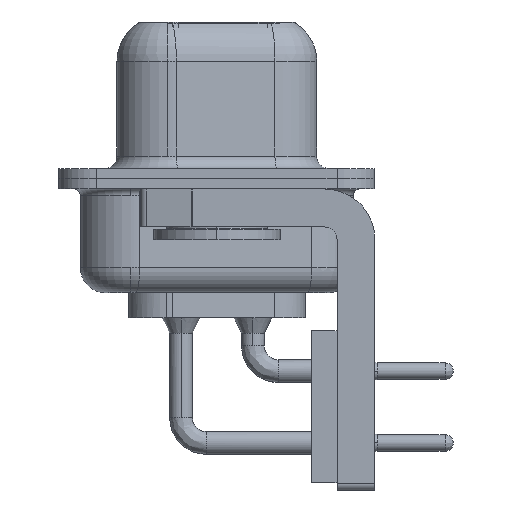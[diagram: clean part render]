
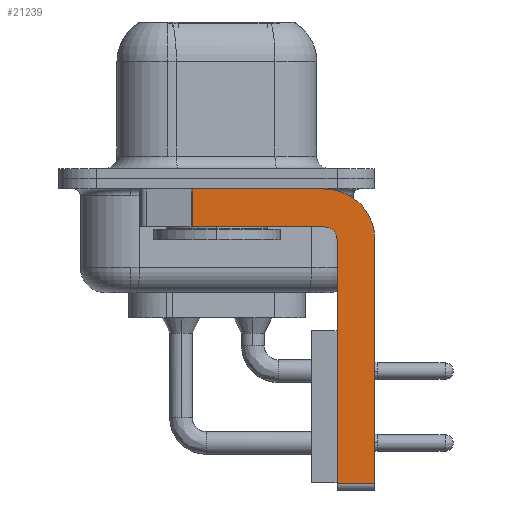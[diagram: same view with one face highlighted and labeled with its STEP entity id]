
A CAD part, left-side view. The second image highlights one B-rep face of the part: STEP entity #21239.
In plain terms, the highlighted planar face has unit normal (-1, 0, 0).
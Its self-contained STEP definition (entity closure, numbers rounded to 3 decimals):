
#61 = EDGE_CURVE ( 'NONE', #13793, #3360, #4816, .T. ) ;
#393 = ORIENTED_EDGE ( 'NONE', *, *, #61, .T. ) ;
#423 = DIRECTION ( 'NONE',  ( 1., 0., 0. ) ) ;
#534 = DIRECTION ( 'NONE',  ( 0., 0., -1. ) ) ;
#1154 = CARTESIAN_POINT ( 'NONE',  ( -2.9, 0.978, -1.9 ) ) ;
#1234 = ORIENTED_EDGE ( 'NONE', *, *, #21657, .F. ) ;
#1652 = CARTESIAN_POINT ( 'NONE',  ( -2.9, -6.25, -12.05 ) ) ;
#1697 = AXIS2_PLACEMENT_3D ( 'NONE', #14634, #2950, #16490 ) ;
#2386 = VECTOR ( 'NONE', #2713, 1000. ) ;
#2548 = VERTEX_POINT ( 'NONE', #20793 ) ;
#2713 = DIRECTION ( 'NONE',  ( 0., 0., 1. ) ) ;
#2915 = CARTESIAN_POINT ( 'NONE',  ( -2.9, -4.25, -1.9 ) ) ;
#2950 = DIRECTION ( 'NONE',  ( -1., 0., 0. ) ) ;
#3360 = VERTEX_POINT ( 'NONE', #1154 ) ;
#3460 = ORIENTED_EDGE ( 'NONE', *, *, #10310, .F. ) ;
#3591 = LINE ( 'NONE', #23923, #2386 ) ;
#4126 = VERTEX_POINT ( 'NONE', #22561 ) ;
#4303 = CARTESIAN_POINT ( 'NONE',  ( -2.9, 0.978, -0.4 ) ) ;
#4647 = VECTOR ( 'NONE', #534, 1000. ) ;
#4730 = EDGE_CURVE ( 'NONE', #20064, #3360, #20481, .T. ) ;
#4816 = LINE ( 'NONE', #22345, #24685 ) ;
#4904 = CARTESIAN_POINT ( 'NONE',  ( -2.9, -4.25, -2.4 ) ) ;
#5040 = VERTEX_POINT ( 'NONE', #22922 ) ;
#5066 = CIRCLE ( 'NONE', #5311, 2. ) ;
#5311 = AXIS2_PLACEMENT_3D ( 'NONE', #12179, #423, #14087 ) ;
#6488 = CARTESIAN_POINT ( 'NONE',  ( -2.9, -4.25, -12.05 ) ) ;
#6624 = VERTEX_POINT ( 'NONE', #19911 ) ;
#6702 = DIRECTION ( 'NONE',  ( 0., 1., 0. ) ) ;
#7469 = CIRCLE ( 'NONE', #1697, 0.5 ) ;
#7531 = ORIENTED_EDGE ( 'NONE', *, *, #8947, .F. ) ;
#8159 = CARTESIAN_POINT ( 'NONE',  ( -2.9, 3., -0.4 ) ) ;
#8947 = EDGE_CURVE ( 'NONE', #4126, #6624, #3591, .T. ) ;
#8955 = DIRECTION ( 'NONE',  ( 0., 0., -1. ) ) ;
#9201 = LINE ( 'NONE', #6488, #18729 ) ;
#9281 = LINE ( 'NONE', #23614, #4647 ) ;
#9599 = AXIS2_PLACEMENT_3D ( 'NONE', #4904, #20341, #8955 ) ;
#10053 = DIRECTION ( 'NONE',  ( 0., 0., -1. ) ) ;
#10310 = EDGE_CURVE ( 'NONE', #5040, #2548, #5066, .T. ) ;
#12132 = FACE_OUTER_BOUND ( 'NONE', #15062, .T. ) ;
#12179 = CARTESIAN_POINT ( 'NONE',  ( -2.9, -4.25, -2.4 ) ) ;
#12372 = DIRECTION ( 'NONE',  ( 0., -1., 0. ) ) ;
#13793 = VERTEX_POINT ( 'NONE', #4303 ) ;
#13887 = LINE ( 'NONE', #8159, #18274 ) ;
#14087 = DIRECTION ( 'NONE',  ( 0., 0., -1. ) ) ;
#14634 = CARTESIAN_POINT ( 'NONE',  ( -2.9, -4.25, -2.4 ) ) ;
#14771 = ORIENTED_EDGE ( 'NONE', *, *, #21184, .F. ) ;
#15062 = EDGE_LOOP ( 'NONE', ( #1234, #393, #21614, #14771, #7531, #24143, #15720, #3460 ) ) ;
#15720 = ORIENTED_EDGE ( 'NONE', *, *, #15893, .F. ) ;
#15893 = EDGE_CURVE ( 'NONE', #2548, #19602, #9281, .T. ) ;
#15897 = DIRECTION ( 'NONE',  ( 0., -1., 0. ) ) ;
#16490 = DIRECTION ( 'NONE',  ( 0., 0., 1. ) ) ;
#17579 = EDGE_CURVE ( 'NONE', #4126, #19602, #9201, .T. ) ;
#18274 = VECTOR ( 'NONE', #15897, 1000. ) ;
#18464 = PLANE ( 'NONE',  #9599 ) ;
#18729 = VECTOR ( 'NONE', #12372, 1000. ) ;
#19602 = VERTEX_POINT ( 'NONE', #1652 ) ;
#19911 = CARTESIAN_POINT ( 'NONE',  ( -2.9, -4.75, -2.4 ) ) ;
#20064 = VERTEX_POINT ( 'NONE', #20222 ) ;
#20222 = CARTESIAN_POINT ( 'NONE',  ( -2.9, -4.25, -1.9 ) ) ;
#20341 = DIRECTION ( 'NONE',  ( 1., 0., 0. ) ) ;
#20481 = LINE ( 'NONE', #2915, #21669 ) ;
#20793 = CARTESIAN_POINT ( 'NONE',  ( -2.9, -6.25, -2.4 ) ) ;
#21184 = EDGE_CURVE ( 'NONE', #6624, #20064, #7469, .T. ) ;
#21239 = ADVANCED_FACE ( 'NONE', ( #12132 ), #18464, .F. ) ;
#21614 = ORIENTED_EDGE ( 'NONE', *, *, #4730, .F. ) ;
#21657 = EDGE_CURVE ( 'NONE', #13793, #5040, #13887, .T. ) ;
#21669 = VECTOR ( 'NONE', #6702, 1000. ) ;
#22345 = CARTESIAN_POINT ( 'NONE',  ( -2.9, 0.978, -1.9 ) ) ;
#22561 = CARTESIAN_POINT ( 'NONE',  ( -2.9, -4.75, -12.05 ) ) ;
#22922 = CARTESIAN_POINT ( 'NONE',  ( -2.9, -4.25, -0.4 ) ) ;
#23614 = CARTESIAN_POINT ( 'NONE',  ( -2.9, -6.25, -2.4 ) ) ;
#23923 = CARTESIAN_POINT ( 'NONE',  ( -2.9, -4.75, -12.3 ) ) ;
#24143 = ORIENTED_EDGE ( 'NONE', *, *, #17579, .T. ) ;
#24685 = VECTOR ( 'NONE', #10053, 1000. ) ;
